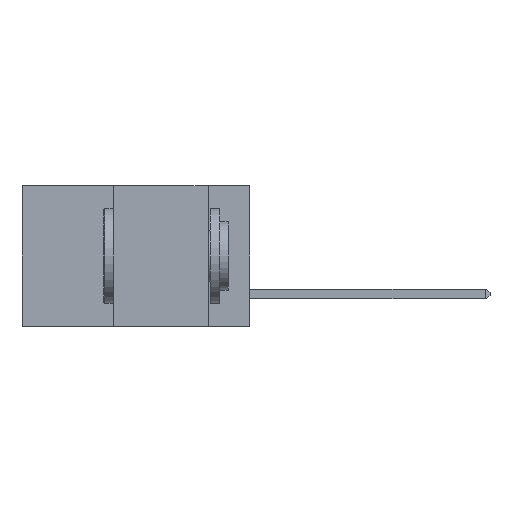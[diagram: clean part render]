
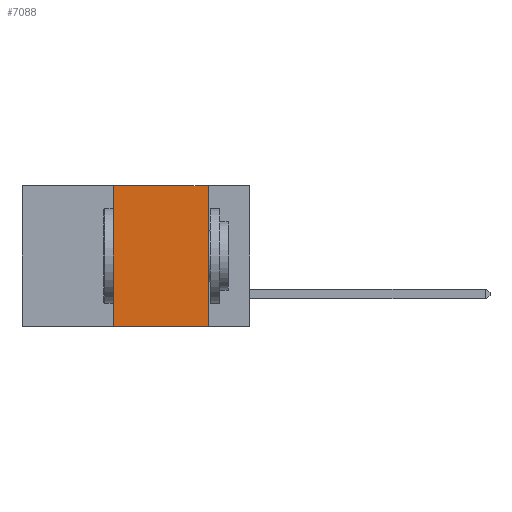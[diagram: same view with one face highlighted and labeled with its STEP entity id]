
A CAD part, left-side view. The second image highlights one B-rep face of the part: STEP entity #7088.
In plain terms, the highlighted planar face has unit normal (-1, 0, 0).
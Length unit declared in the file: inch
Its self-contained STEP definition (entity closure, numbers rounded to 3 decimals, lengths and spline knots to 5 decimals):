
#977 = PLANE ( 'NONE',  #5583 ) ;
#1026 = ORIENTED_EDGE ( 'NONE', *, *, #1214, .F. ) ;
#1214 = EDGE_CURVE ( 'NONE', #2673, #7307, #10899, .T. ) ;
#2028 = CARTESIAN_POINT ( 'NONE',  ( 0., 0.6, 0. ) ) ;
#2350 = ORIENTED_EDGE ( 'NONE', *, *, #2395, .T. ) ;
#2395 = EDGE_CURVE ( 'NONE', #10041, #7307, #9654, .T. ) ;
#2673 = VERTEX_POINT ( 'NONE', #9958 ) ;
#3084 = DIRECTION ( 'NONE',  ( 0., 0., -1. ) ) ;
#3140 = LINE ( 'NONE', #11477, #7817 ) ;
#3162 = CARTESIAN_POINT ( 'NONE',  ( 0., 0.36, 0. ) ) ;
#3476 = VERTEX_POINT ( 'NONE', #3162 ) ;
#4372 = CARTESIAN_POINT ( 'NONE',  ( 0., 0.11, -0.37 ) ) ;
#4851 = EDGE_LOOP ( 'NONE', ( #1026, #9118, #6751, #2350 ) ) ;
#5163 = EDGE_CURVE ( 'NONE', #3476, #2673, #10677, .T. ) ;
#5455 = CARTESIAN_POINT ( 'NONE',  ( 0., 0.11, 0. ) ) ;
#5537 = DIRECTION ( 'NONE',  ( 0., 0., -1. ) ) ;
#5583 = AXIS2_PLACEMENT_3D ( 'NONE', #2028, #9085, #3084 ) ;
#5714 = EDGE_CURVE ( 'NONE', #10041, #3476, #3140, .T. ) ;
#6674 = VECTOR ( 'NONE', #12059, 39.37008 ) ;
#6751 = ORIENTED_EDGE ( 'NONE', *, *, #5714, .F. ) ;
#7008 = CARTESIAN_POINT ( 'NONE',  ( 0., 0.36, -0.37 ) ) ;
#7088 = ADVANCED_FACE ( 'NONE', ( #9513 ), #977, .F. ) ;
#7307 = VERTEX_POINT ( 'NONE', #4372 ) ;
#7711 = VECTOR ( 'NONE', #9099, 39.37008 ) ;
#7817 = VECTOR ( 'NONE', #8579, 39.37008 ) ;
#8263 = VECTOR ( 'NONE', #5537, 39.37008 ) ;
#8579 = DIRECTION ( 'NONE',  ( 0., 0., 1. ) ) ;
#8996 = CARTESIAN_POINT ( 'NONE',  ( 0., 0.6, 0. ) ) ;
#9085 = DIRECTION ( 'NONE',  ( 1., 0., 0. ) ) ;
#9099 = DIRECTION ( 'NONE',  ( 0., -1., 0. ) ) ;
#9118 = ORIENTED_EDGE ( 'NONE', *, *, #5163, .F. ) ;
#9513 = FACE_OUTER_BOUND ( 'NONE', #4851, .T. ) ;
#9654 = LINE ( 'NONE', #12442, #6674 ) ;
#9958 = CARTESIAN_POINT ( 'NONE',  ( 0., 0.11, 0. ) ) ;
#10041 = VERTEX_POINT ( 'NONE', #7008 ) ;
#10677 = LINE ( 'NONE', #8996, #7711 ) ;
#10899 = LINE ( 'NONE', #5455, #8263 ) ;
#11477 = CARTESIAN_POINT ( 'NONE',  ( 0., 0.36, 0. ) ) ;
#12059 = DIRECTION ( 'NONE',  ( 0., -1., 0. ) ) ;
#12442 = CARTESIAN_POINT ( 'NONE',  ( 0., 0.6, -0.37 ) ) ;
